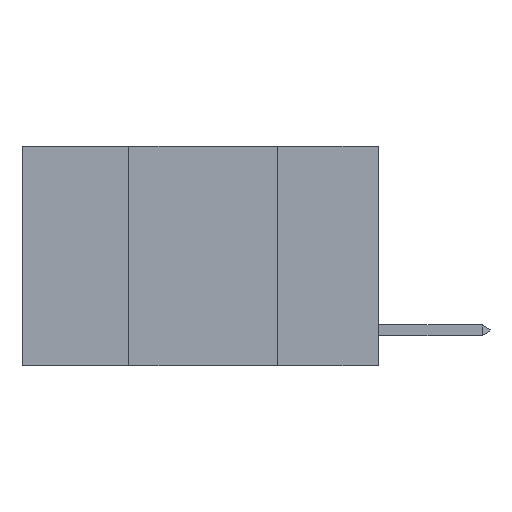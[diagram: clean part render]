
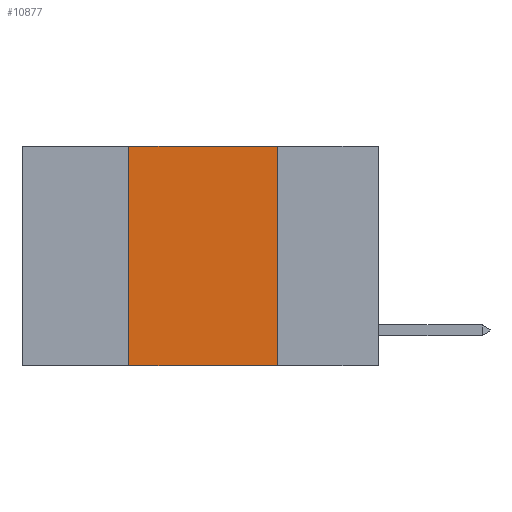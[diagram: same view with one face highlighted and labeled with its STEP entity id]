
A CAD part, left-side view. The second image highlights one B-rep face of the part: STEP entity #10877.
In plain terms, the highlighted planar face has unit normal (-1, 0, 0).
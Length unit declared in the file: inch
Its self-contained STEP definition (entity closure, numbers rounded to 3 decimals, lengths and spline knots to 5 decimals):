
#734 = LINE ( 'NONE', #23474, #4236 ) ;
#1711 = DIRECTION ( 'NONE',  ( 1., 0., 0. ) ) ;
#1782 = DIRECTION ( 'NONE',  ( 0., -1., 0. ) ) ;
#2043 = CARTESIAN_POINT ( 'NONE',  ( 0., 0.6, 0. ) ) ;
#3258 = CARTESIAN_POINT ( 'NONE',  ( 0., 0.42, 0. ) ) ;
#3450 = AXIS2_PLACEMENT_3D ( 'NONE', #17718, #1711, #19875 ) ;
#4205 = CARTESIAN_POINT ( 'NONE',  ( 0., 0.6, -0.37 ) ) ;
#4236 = VECTOR ( 'NONE', #8984, 39.37008 ) ;
#8531 = EDGE_CURVE ( 'NONE', #24281, #16154, #734, .T. ) ;
#8664 = EDGE_CURVE ( 'NONE', #21615, #12718, #26300, .T. ) ;
#8984 = DIRECTION ( 'NONE',  ( 0., 0., 1. ) ) ;
#10306 = VECTOR ( 'NONE', #15756, 39.37008 ) ;
#10455 = DIRECTION ( 'NONE',  ( 0., -1., 0. ) ) ;
#10877 = ADVANCED_FACE ( 'NONE', ( #13764 ), #21870, .F. ) ;
#11942 = LINE ( 'NONE', #2043, #20167 ) ;
#12718 = VERTEX_POINT ( 'NONE', #22814 ) ;
#13719 = CARTESIAN_POINT ( 'NONE',  ( 0., 0.17, 0. ) ) ;
#13764 = FACE_OUTER_BOUND ( 'NONE', #24766, .T. ) ;
#14776 = ORIENTED_EDGE ( 'NONE', *, *, #16174, .T. ) ;
#15756 = DIRECTION ( 'NONE',  ( 0., 0., -1. ) ) ;
#15889 = CARTESIAN_POINT ( 'NONE',  ( 0., 0.42, -0.37 ) ) ;
#16154 = VERTEX_POINT ( 'NONE', #3258 ) ;
#16174 = EDGE_CURVE ( 'NONE', #24281, #12718, #22754, .T. ) ;
#16240 = EDGE_CURVE ( 'NONE', #16154, #21615, #11942, .T. ) ;
#17718 = CARTESIAN_POINT ( 'NONE',  ( 0., 0.6, 0. ) ) ;
#18138 = ORIENTED_EDGE ( 'NONE', *, *, #8531, .F. ) ;
#19875 = DIRECTION ( 'NONE',  ( 0., 0., -1. ) ) ;
#20167 = VECTOR ( 'NONE', #1782, 39.37008 ) ;
#21615 = VERTEX_POINT ( 'NONE', #26400 ) ;
#21870 = PLANE ( 'NONE',  #3450 ) ;
#22737 = VECTOR ( 'NONE', #10455, 39.37008 ) ;
#22754 = LINE ( 'NONE', #4205, #22737 ) ;
#22814 = CARTESIAN_POINT ( 'NONE',  ( 0., 0.17, -0.37 ) ) ;
#23474 = CARTESIAN_POINT ( 'NONE',  ( 0., 0.42, 0. ) ) ;
#24281 = VERTEX_POINT ( 'NONE', #15889 ) ;
#24535 = ORIENTED_EDGE ( 'NONE', *, *, #16240, .F. ) ;
#24766 = EDGE_LOOP ( 'NONE', ( #25541, #24535, #18138, #14776 ) ) ;
#25541 = ORIENTED_EDGE ( 'NONE', *, *, #8664, .F. ) ;
#26300 = LINE ( 'NONE', #13719, #10306 ) ;
#26400 = CARTESIAN_POINT ( 'NONE',  ( 0., 0.17, 0. ) ) ;
